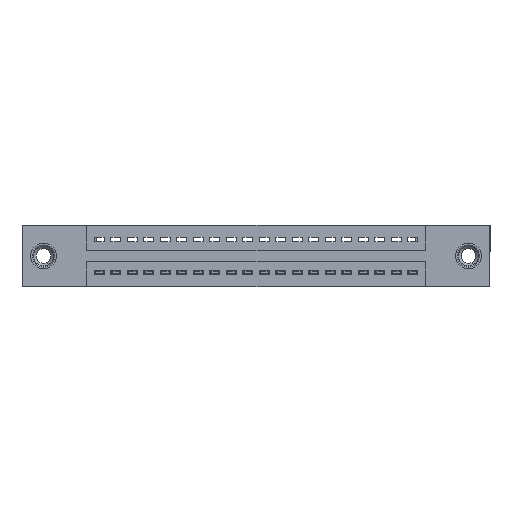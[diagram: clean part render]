
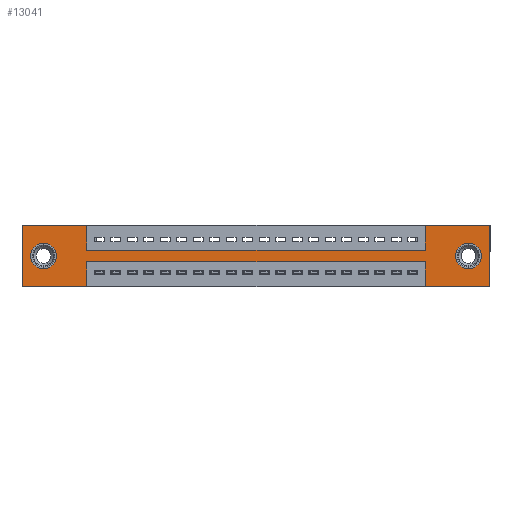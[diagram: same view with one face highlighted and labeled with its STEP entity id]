
A CAD part, front view. The second image highlights one B-rep face of the part: STEP entity #13041.
In plain terms, the highlighted planar face has unit normal (0, -1, 0).
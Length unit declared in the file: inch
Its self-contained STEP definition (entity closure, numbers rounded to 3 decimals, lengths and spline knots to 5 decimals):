
#28 = VECTOR ( 'NONE', #13417, 39.37008 ) ;
#130 = VECTOR ( 'NONE', #7404, 39.37008 ) ;
#165 = VERTEX_POINT ( 'NONE', #13398 ) ;
#196 = EDGE_CURVE ( 'NONE', #16621, #5586, #17977, .T. ) ;
#287 = LINE ( 'NONE', #14548, #7271 ) ;
#467 = EDGE_CURVE ( 'NONE', #165, #6152, #5644, .T. ) ;
#530 = CIRCLE ( 'NONE', #17642, 0.078 ) ;
#596 = DIRECTION ( 'NONE',  ( 0., 0., -1. ) ) ;
#657 = CARTESIAN_POINT ( 'NONE',  ( 0., 0., 0. ) ) ;
#694 = CARTESIAN_POINT ( 'NONE',  ( 0.3925, 0., -0.22 ) ) ;
#719 = DIRECTION ( 'NONE',  ( 0., 0., 1. ) ) ;
#1248 = VECTOR ( 'NONE', #16179, 39.37008 ) ;
#1555 = EDGE_CURVE ( 'NONE', #10581, #165, #14517, .T. ) ;
#1647 = ORIENTED_EDGE ( 'NONE', *, *, #18771, .F. ) ;
#1805 = DIRECTION ( 'NONE',  ( 0., 0., 1. ) ) ;
#2081 = CIRCLE ( 'NONE', #15431, 0.078 ) ;
#2427 = LINE ( 'NONE', #3210, #3398 ) ;
#2556 = AXIS2_PLACEMENT_3D ( 'NONE', #17103, #18871, #1805 ) ;
#3126 = VERTEX_POINT ( 'NONE', #6049 ) ;
#3210 = CARTESIAN_POINT ( 'NONE',  ( 2.4425, 0., -0.37 ) ) ;
#3241 = DIRECTION ( 'NONE',  ( 0., 1., 0. ) ) ;
#3398 = VECTOR ( 'NONE', #15799, 39.37008 ) ;
#3508 = EDGE_CURVE ( 'NONE', #9522, #16503, #16331, .T. ) ;
#3906 = VERTEX_POINT ( 'NONE', #6120 ) ;
#3924 = CARTESIAN_POINT ( 'NONE',  ( 2.705, 0., -0.263 ) ) ;
#3998 = ORIENTED_EDGE ( 'NONE', *, *, #12261, .T. ) ;
#4338 = ORIENTED_EDGE ( 'NONE', *, *, #196, .F. ) ;
#4597 = DIRECTION ( 'NONE',  ( 0., 0., -1. ) ) ;
#4812 = ORIENTED_EDGE ( 'NONE', *, *, #14357, .F. ) ;
#4961 = CARTESIAN_POINT ( 'NONE',  ( 0., 0., 0. ) ) ;
#5048 = CARTESIAN_POINT ( 'NONE',  ( 0.13, 0., -0.185 ) ) ;
#5202 = PLANE ( 'NONE',  #14041 ) ;
#5433 = DIRECTION ( 'NONE',  ( -1., 0., 0. ) ) ;
#5586 = VERTEX_POINT ( 'NONE', #16326 ) ;
#5644 = LINE ( 'NONE', #11662, #16755 ) ;
#5879 = CARTESIAN_POINT ( 'NONE',  ( 0.3925, 0., -0.15 ) ) ;
#5958 = CARTESIAN_POINT ( 'NONE',  ( 0.3925, 0., -0.37 ) ) ;
#6049 = CARTESIAN_POINT ( 'NONE',  ( 0.13, 0., -0.107 ) ) ;
#6120 = CARTESIAN_POINT ( 'NONE',  ( 2.4425, 0., -0.37 ) ) ;
#6152 = VERTEX_POINT ( 'NONE', #13123 ) ;
#6254 = LINE ( 'NONE', #18219, #28 ) ;
#6271 = CIRCLE ( 'NONE', #6965, 0.078 ) ;
#6326 = DIRECTION ( 'NONE',  ( 0., 0., 1. ) ) ;
#6350 = CARTESIAN_POINT ( 'NONE',  ( 0.13, 0., -0.263 ) ) ;
#6501 = CARTESIAN_POINT ( 'NONE',  ( 0.3925, 0., 0. ) ) ;
#6531 = ORIENTED_EDGE ( 'NONE', *, *, #12929, .T. ) ;
#6602 = VERTEX_POINT ( 'NONE', #8102 ) ;
#6817 = EDGE_CURVE ( 'NONE', #6152, #9522, #17920, .T. ) ;
#6821 = ORIENTED_EDGE ( 'NONE', *, *, #16639, .F. ) ;
#6965 = AXIS2_PLACEMENT_3D ( 'NONE', #12490, #3241, #7736 ) ;
#7245 = LINE ( 'NONE', #6501, #14016 ) ;
#7271 = VECTOR ( 'NONE', #16113, 39.37008 ) ;
#7401 = VERTEX_POINT ( 'NONE', #3924 ) ;
#7404 = DIRECTION ( 'NONE',  ( 1., 0., 0. ) ) ;
#7441 = ORIENTED_EDGE ( 'NONE', *, *, #1555, .F. ) ;
#7514 = DIRECTION ( 'NONE',  ( 0., 0., -1. ) ) ;
#7599 = EDGE_LOOP ( 'NONE', ( #3998, #6531 ) ) ;
#7736 = DIRECTION ( 'NONE',  ( 0., 0., -1. ) ) ;
#8047 = CARTESIAN_POINT ( 'NONE',  ( 2.705, 0., -0.185 ) ) ;
#8102 = CARTESIAN_POINT ( 'NONE',  ( 2.4425, 0., -0.15 ) ) ;
#8131 = LINE ( 'NONE', #12775, #18769 ) ;
#8456 = LINE ( 'NONE', #694, #1248 ) ;
#9522 = VERTEX_POINT ( 'NONE', #4961 ) ;
#9537 = DIRECTION ( 'NONE',  ( 0., 0., -1. ) ) ;
#9755 = EDGE_CURVE ( 'NONE', #7401, #19494, #2081, .T. ) ;
#9914 = FACE_OUTER_BOUND ( 'NONE', #12559, .T. ) ;
#10288 = VERTEX_POINT ( 'NONE', #14178 ) ;
#10356 = CARTESIAN_POINT ( 'NONE',  ( 2.835, 0., -0.37 ) ) ;
#10581 = VERTEX_POINT ( 'NONE', #19376 ) ;
#10666 = ORIENTED_EDGE ( 'NONE', *, *, #13293, .F. ) ;
#10766 = DIRECTION ( 'NONE',  ( 0., 1., 0. ) ) ;
#10847 = CARTESIAN_POINT ( 'NONE',  ( 0., 0., 0. ) ) ;
#10984 = VECTOR ( 'NONE', #18105, 39.37008 ) ;
#11372 = CARTESIAN_POINT ( 'NONE',  ( 0., 0., -0.37 ) ) ;
#11662 = CARTESIAN_POINT ( 'NONE',  ( 0., 0., -0.37 ) ) ;
#11865 = FACE_BOUND ( 'NONE', #7599, .T. ) ;
#12251 = ORIENTED_EDGE ( 'NONE', *, *, #467, .F. ) ;
#12261 = EDGE_CURVE ( 'NONE', #3126, #13412, #530, .T. ) ;
#12412 = DIRECTION ( 'NONE',  ( 1., 0., 0. ) ) ;
#12490 = CARTESIAN_POINT ( 'NONE',  ( 2.705, 0., -0.185 ) ) ;
#12559 = EDGE_LOOP ( 'NONE', ( #7441, #16575, #10666, #6821, #16690, #4338, #1647, #4812, #13243, #14714, #18187, #12251 ) ) ;
#12775 = CARTESIAN_POINT ( 'NONE',  ( 2.4425, 0., 0. ) ) ;
#12869 = DIRECTION ( 'NONE',  ( 0., -1., 0. ) ) ;
#12929 = EDGE_CURVE ( 'NONE', #13412, #3126, #13530, .T. ) ;
#13041 = ADVANCED_FACE ( 'NONE', ( #16438, #11865, #9914 ), #5202, .T. ) ;
#13123 = CARTESIAN_POINT ( 'NONE',  ( 0., 0., -0.37 ) ) ;
#13243 = ORIENTED_EDGE ( 'NONE', *, *, #16940, .F. ) ;
#13293 = EDGE_CURVE ( 'NONE', #3906, #10288, #2427, .T. ) ;
#13398 = CARTESIAN_POINT ( 'NONE',  ( 0.3925, 0., -0.37 ) ) ;
#13412 = VERTEX_POINT ( 'NONE', #6350 ) ;
#13417 = DIRECTION ( 'NONE',  ( 0., 0., -1. ) ) ;
#13469 = CARTESIAN_POINT ( 'NONE',  ( 0., 0., 0. ) ) ;
#13530 = CIRCLE ( 'NONE', #2556, 0.078 ) ;
#13927 = VECTOR ( 'NONE', #12412, 39.37008 ) ;
#14016 = VECTOR ( 'NONE', #9537, 39.37008 ) ;
#14041 = AXIS2_PLACEMENT_3D ( 'NONE', #11372, #12869, #596 ) ;
#14178 = CARTESIAN_POINT ( 'NONE',  ( 2.4425, 0., -0.22 ) ) ;
#14357 = EDGE_CURVE ( 'NONE', #16384, #6602, #19204, .T. ) ;
#14517 = LINE ( 'NONE', #5958, #18888 ) ;
#14548 = CARTESIAN_POINT ( 'NONE',  ( 0., 0., -0.37 ) ) ;
#14714 = ORIENTED_EDGE ( 'NONE', *, *, #3508, .F. ) ;
#15207 = ORIENTED_EDGE ( 'NONE', *, *, #16309, .T. ) ;
#15421 = VERTEX_POINT ( 'NONE', #10356 ) ;
#15431 = AXIS2_PLACEMENT_3D ( 'NONE', #8047, #10766, #4597 ) ;
#15781 = EDGE_CURVE ( 'NONE', #10288, #10581, #8456, .T. ) ;
#15799 = DIRECTION ( 'NONE',  ( 0., 0., 1. ) ) ;
#15852 = DIRECTION ( 'NONE',  ( 0., 1., 0. ) ) ;
#16113 = DIRECTION ( 'NONE',  ( -1., 0., 0. ) ) ;
#16165 = EDGE_LOOP ( 'NONE', ( #15207, #18596 ) ) ;
#16179 = DIRECTION ( 'NONE',  ( -1., 0., 0. ) ) ;
#16309 = EDGE_CURVE ( 'NONE', #19494, #7401, #6271, .T. ) ;
#16326 = CARTESIAN_POINT ( 'NONE',  ( 2.835, 0., 0. ) ) ;
#16331 = LINE ( 'NONE', #10847, #13927 ) ;
#16384 = VERTEX_POINT ( 'NONE', #5879 ) ;
#16438 = FACE_BOUND ( 'NONE', #16165, .T. ) ;
#16503 = VERTEX_POINT ( 'NONE', #16827 ) ;
#16543 = CARTESIAN_POINT ( 'NONE',  ( 0.3925, 0., -0.15 ) ) ;
#16575 = ORIENTED_EDGE ( 'NONE', *, *, #15781, .F. ) ;
#16621 = VERTEX_POINT ( 'NONE', #17466 ) ;
#16639 = EDGE_CURVE ( 'NONE', #15421, #3906, #287, .T. ) ;
#16690 = ORIENTED_EDGE ( 'NONE', *, *, #17229, .F. ) ;
#16755 = VECTOR ( 'NONE', #5433, 39.37008 ) ;
#16827 = CARTESIAN_POINT ( 'NONE',  ( 0.3925, 0., 0. ) ) ;
#16940 = EDGE_CURVE ( 'NONE', #16503, #16384, #7245, .T. ) ;
#17103 = CARTESIAN_POINT ( 'NONE',  ( 0.13, 0., -0.185 ) ) ;
#17216 = DIRECTION ( 'NONE',  ( 0., 0., 1. ) ) ;
#17229 = EDGE_CURVE ( 'NONE', #5586, #15421, #6254, .T. ) ;
#17466 = CARTESIAN_POINT ( 'NONE',  ( 2.4425, 0., 0. ) ) ;
#17642 = AXIS2_PLACEMENT_3D ( 'NONE', #5048, #15852, #6326 ) ;
#17920 = LINE ( 'NONE', #657, #19637 ) ;
#17977 = LINE ( 'NONE', #13469, #130 ) ;
#18105 = DIRECTION ( 'NONE',  ( 1., 0., 0. ) ) ;
#18187 = ORIENTED_EDGE ( 'NONE', *, *, #6817, .F. ) ;
#18219 = CARTESIAN_POINT ( 'NONE',  ( 2.835, 0., 0. ) ) ;
#18596 = ORIENTED_EDGE ( 'NONE', *, *, #9755, .T. ) ;
#18769 = VECTOR ( 'NONE', #17216, 39.37008 ) ;
#18771 = EDGE_CURVE ( 'NONE', #6602, #16621, #8131, .T. ) ;
#18871 = DIRECTION ( 'NONE',  ( 0., 1., 0. ) ) ;
#18888 = VECTOR ( 'NONE', #7514, 39.37008 ) ;
#19095 = CARTESIAN_POINT ( 'NONE',  ( 2.705, 0., -0.107 ) ) ;
#19204 = LINE ( 'NONE', #16543, #10984 ) ;
#19376 = CARTESIAN_POINT ( 'NONE',  ( 0.3925, 0., -0.22 ) ) ;
#19494 = VERTEX_POINT ( 'NONE', #19095 ) ;
#19637 = VECTOR ( 'NONE', #719, 39.37008 ) ;
